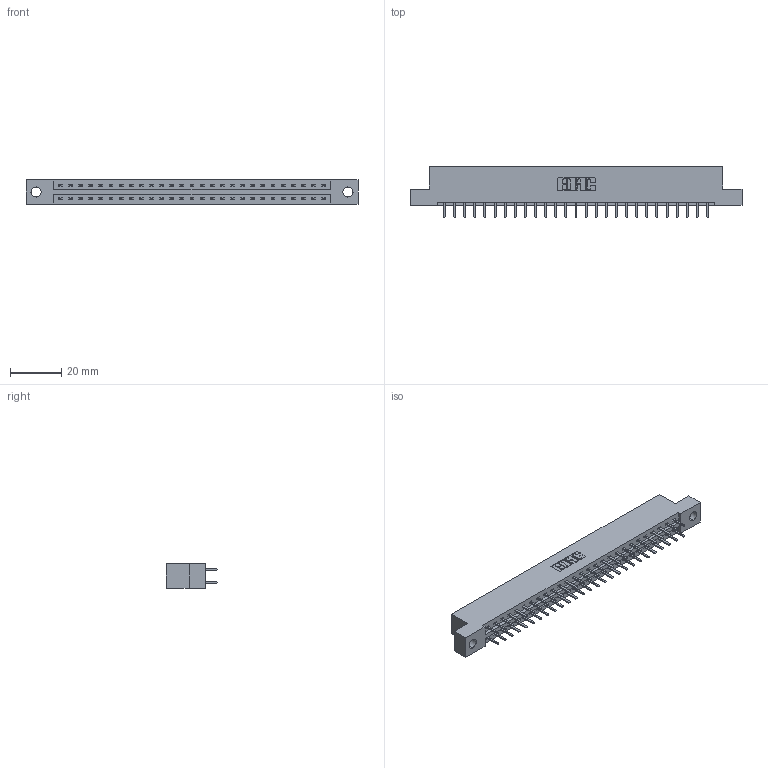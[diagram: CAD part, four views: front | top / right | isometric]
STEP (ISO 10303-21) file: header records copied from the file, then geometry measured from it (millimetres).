
FILE_DESCRIPTION (( 'STEP AP203' ), '1' );
FILE_NAME ('337-054-520-204.STEP', '2018-08-10T00:06:20', ( '' ), ( '' ), 'SwSTEP 2.0', 'SolidWorks 2016', '' );
FILE_SCHEMA (( 'CONFIG_CONTROL_DESIGN' ));
Length unit declared in the file: inch
Products named in the file (3): 337 Part_Flush Mounting Lugs - 0.156 Dia-TH; 345-292-001_345-293-120; 337-054-520-204
Assembly tree (55 placements, depth 2):
  337-054-520-204
    337 Part_Flush Mounting Lugs - 0.156 Dia-TH
    345-292-001_345-293-120  x54
Bounding box: 130 x 20.02 x 9.4 mm (x, y, z)
Volume: 13388.9 mm3; surface area: 14720.1 mm2
Topology: 55 solids, 55 shells, 3246 faces, 9437 edges, 6146 vertices
Faces by surface type: plane 2230, cylinder 1016
Entity records: 22991 total; most frequent: CARTESIAN_POINT 3898, ORIENTED_EDGE 3822, DIRECTION 3331, EDGE_CURVE 1911, VECTOR 1779, LINE 1779, VERTEX_POINT 1270, AXIS2_PLACEMENT_3D 776
